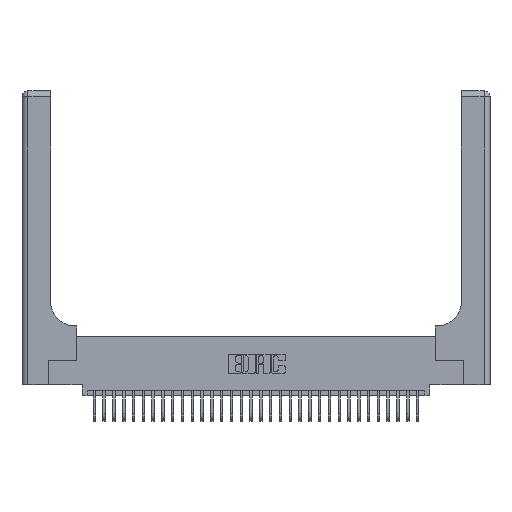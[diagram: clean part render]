
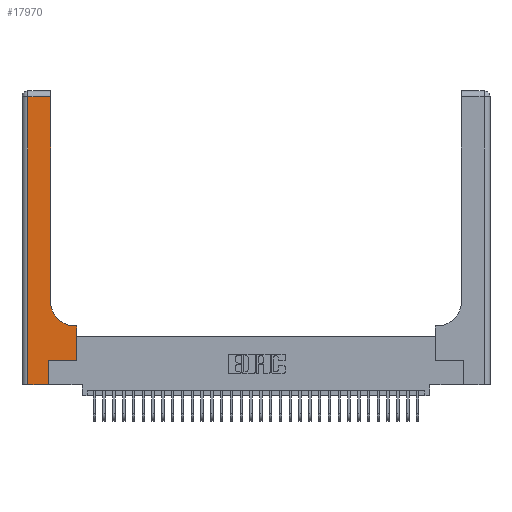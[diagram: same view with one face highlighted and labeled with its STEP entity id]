
A CAD part, top view. The second image highlights one B-rep face of the part: STEP entity #17970.
In plain terms, the highlighted planar face has unit normal (0, 0, 1).
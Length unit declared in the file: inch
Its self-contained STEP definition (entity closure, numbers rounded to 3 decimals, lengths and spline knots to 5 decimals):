
#1402 = CARTESIAN_POINT ( 'NONE',  ( 0.269, 0.25, 0.37 ) ) ;
#1740 = CARTESIAN_POINT ( 'NONE',  ( 0.5585, 0.25, 0.37 ) ) ;
#1978 = VERTEX_POINT ( 'NONE', #4877 ) ;
#2699 = ORIENTED_EDGE ( 'NONE', *, *, #23786, .T. ) ;
#2700 = AXIS2_PLACEMENT_3D ( 'NONE', #23619, #6303, #23725 ) ;
#2813 = EDGE_CURVE ( 'NONE', #15421, #28525, #24711, .T. ) ;
#2934 = CARTESIAN_POINT ( 'NONE',  ( 0.5415, 0.85, 0.37 ) ) ;
#3682 = VERTEX_POINT ( 'NONE', #8347 ) ;
#4857 = AXIS2_PLACEMENT_3D ( 'NONE', #2934, #20344, #5433 ) ;
#4877 = CARTESIAN_POINT ( 'NONE',  ( 0.5415, 0.6, 0.37 ) ) ;
#5433 = DIRECTION ( 'NONE',  ( 1., 0., 0. ) ) ;
#5597 = DIRECTION ( 'NONE',  ( -1., 0., 0. ) ) ;
#6072 = FACE_OUTER_BOUND ( 'NONE', #7756, .T. ) ;
#6303 = DIRECTION ( 'NONE',  ( 0., 0., -1. ) ) ;
#6339 = VECTOR ( 'NONE', #5597, 39.37008 ) ;
#6467 = LINE ( 'NONE', #23390, #25519 ) ;
#6885 = EDGE_CURVE ( 'NONE', #1978, #15421, #29618, .T. ) ;
#7756 = EDGE_LOOP ( 'NONE', ( #10413, #12078, #13682, #17311, #10839, #15536, #2699, #30599, #11275 ) ) ;
#7871 = LINE ( 'NONE', #25368, #6339 ) ;
#8139 = VECTOR ( 'NONE', #18569, 39.37008 ) ;
#8347 = CARTESIAN_POINT ( 'NONE',  ( 0.06, 0., 0.37 ) ) ;
#8355 = LINE ( 'NONE', #10939, #21635 ) ;
#9052 = CARTESIAN_POINT ( 'NONE',  ( 0.06, 2.94, 0.37 ) ) ;
#9867 = VECTOR ( 'NONE', #15518, 39.37008 ) ;
#10042 = DIRECTION ( 'NONE',  ( 1., 0., 0. ) ) ;
#10186 = EDGE_CURVE ( 'NONE', #23355, #28579, #31290, .T. ) ;
#10413 = ORIENTED_EDGE ( 'NONE', *, *, #2813, .T. ) ;
#10490 = CARTESIAN_POINT ( 'NONE',  ( 0.5585, 0.25, 0.37 ) ) ;
#10839 = ORIENTED_EDGE ( 'NONE', *, *, #15928, .T. ) ;
#10939 = CARTESIAN_POINT ( 'NONE',  ( 0.06, 3., 0.37 ) ) ;
#11082 = EDGE_CURVE ( 'NONE', #3682, #25009, #6467, .T. ) ;
#11275 = ORIENTED_EDGE ( 'NONE', *, *, #6885, .T. ) ;
#12078 = ORIENTED_EDGE ( 'NONE', *, *, #29504, .T. ) ;
#12094 = DIRECTION ( 'NONE',  ( -1., 0., 0. ) ) ;
#12423 = CARTESIAN_POINT ( 'NONE',  ( 0.269, 0.25, 0.37 ) ) ;
#12907 = EDGE_CURVE ( 'NONE', #22506, #3682, #8355, .T. ) ;
#13522 = CARTESIAN_POINT ( 'NONE',  ( 0.2915, 3., 0.37 ) ) ;
#13682 = ORIENTED_EDGE ( 'NONE', *, *, #12907, .T. ) ;
#13702 = PLANE ( 'NONE',  #2700 ) ;
#14639 = VECTOR ( 'NONE', #12094, 39.37008 ) ;
#15421 = VERTEX_POINT ( 'NONE', #21858 ) ;
#15518 = DIRECTION ( 'NONE',  ( 0., 1., 0. ) ) ;
#15536 = ORIENTED_EDGE ( 'NONE', *, *, #10186, .T. ) ;
#15928 = EDGE_CURVE ( 'NONE', #25009, #23355, #27979, .T. ) ;
#16526 = LINE ( 'NONE', #10490, #9867 ) ;
#17052 = CARTESIAN_POINT ( 'NONE',  ( 0.2915, 0.6, 0.37 ) ) ;
#17311 = ORIENTED_EDGE ( 'NONE', *, *, #11082, .T. ) ;
#17970 = ADVANCED_FACE ( 'NONE', ( #6072 ), #13702, .F. ) ;
#18249 = VECTOR ( 'NONE', #10042, 39.37008 ) ;
#18569 = DIRECTION ( 'NONE',  ( 0., 1., 0. ) ) ;
#18724 = CARTESIAN_POINT ( 'NONE',  ( 0.269, 0., 0.37 ) ) ;
#18887 = VECTOR ( 'NONE', #30774, 39.37008 ) ;
#20344 = DIRECTION ( 'NONE',  ( 0., 0., -1. ) ) ;
#20931 = CARTESIAN_POINT ( 'NONE',  ( 0.2915, 2.94, 0.37 ) ) ;
#21635 = VECTOR ( 'NONE', #28311, 39.37008 ) ;
#21858 = CARTESIAN_POINT ( 'NONE',  ( 0.2915, 0.85, 0.37 ) ) ;
#22506 = VERTEX_POINT ( 'NONE', #9052 ) ;
#22664 = EDGE_CURVE ( 'NONE', #31797, #1978, #22823, .T. ) ;
#22823 = LINE ( 'NONE', #17052, #14639 ) ;
#23355 = VERTEX_POINT ( 'NONE', #1402 ) ;
#23390 = CARTESIAN_POINT ( 'NONE',  ( 0., 0., 0.37 ) ) ;
#23449 = CARTESIAN_POINT ( 'NONE',  ( 0.5585, 0.6, 0.37 ) ) ;
#23619 = CARTESIAN_POINT ( 'NONE',  ( 0., 3., 0.37 ) ) ;
#23725 = DIRECTION ( 'NONE',  ( -1., 0., 0. ) ) ;
#23786 = EDGE_CURVE ( 'NONE', #28579, #31797, #16526, .T. ) ;
#24711 = LINE ( 'NONE', #13522, #18887 ) ;
#25009 = VERTEX_POINT ( 'NONE', #18724 ) ;
#25368 = CARTESIAN_POINT ( 'NONE',  ( 0., 2.94, 0.37 ) ) ;
#25519 = VECTOR ( 'NONE', #25871, 39.37008 ) ;
#25871 = DIRECTION ( 'NONE',  ( 1., 0., 0. ) ) ;
#27979 = LINE ( 'NONE', #30786, #8139 ) ;
#28311 = DIRECTION ( 'NONE',  ( 0., -1., 0. ) ) ;
#28525 = VERTEX_POINT ( 'NONE', #20931 ) ;
#28579 = VERTEX_POINT ( 'NONE', #1740 ) ;
#29504 = EDGE_CURVE ( 'NONE', #28525, #22506, #7871, .T. ) ;
#29618 = CIRCLE ( 'NONE', #4857, 0.25 ) ;
#30599 = ORIENTED_EDGE ( 'NONE', *, *, #22664, .T. ) ;
#30774 = DIRECTION ( 'NONE',  ( 0., 1., 0. ) ) ;
#30786 = CARTESIAN_POINT ( 'NONE',  ( 0.269, 0., 0.37 ) ) ;
#31290 = LINE ( 'NONE', #12423, #18249 ) ;
#31797 = VERTEX_POINT ( 'NONE', #23449 ) ;
